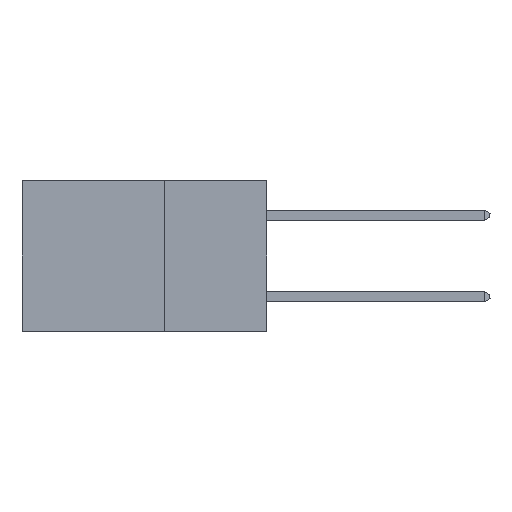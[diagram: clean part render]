
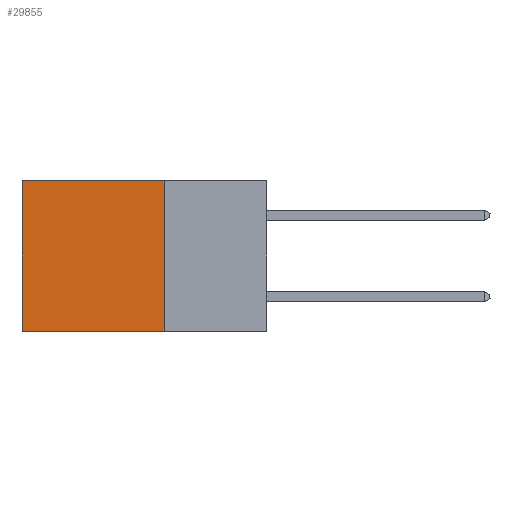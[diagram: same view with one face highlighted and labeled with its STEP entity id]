
A CAD part, left-side view. The second image highlights one B-rep face of the part: STEP entity #29855.
In plain terms, the highlighted planar face has unit normal (-1, 0, 0).
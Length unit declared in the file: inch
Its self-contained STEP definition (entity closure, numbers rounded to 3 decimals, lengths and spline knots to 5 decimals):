
#562 = LINE ( 'NONE', #22025, #26445 ) ;
#1648 = EDGE_CURVE ( 'NONE', #13397, #27911, #10706, .T. ) ;
#1981 = VECTOR ( 'NONE', #32892, 39.37008 ) ;
#3387 = DIRECTION ( 'NONE',  ( 0., 0., -1. ) ) ;
#3437 = CARTESIAN_POINT ( 'NONE',  ( 0.2875, 0.25, 0. ) ) ;
#3974 = DIRECTION ( 'NONE',  ( 0., 1., 0. ) ) ;
#5777 = DIRECTION ( 'NONE',  ( 0., 0., -1. ) ) ;
#6003 = ORIENTED_EDGE ( 'NONE', *, *, #9754, .T. ) ;
#8329 = DIRECTION ( 'NONE',  ( 1., 0., 0. ) ) ;
#9754 = EDGE_CURVE ( 'NONE', #31652, #13397, #562, .T. ) ;
#9827 = CARTESIAN_POINT ( 'NONE',  ( 0.2875, 0.25, -0.37 ) ) ;
#10706 = LINE ( 'NONE', #31030, #23115 ) ;
#11102 = EDGE_CURVE ( 'NONE', #31652, #31467, #21652, .T. ) ;
#11314 = CARTESIAN_POINT ( 'NONE',  ( 0.2875, 0.25, 0. ) ) ;
#12085 = CARTESIAN_POINT ( 'NONE',  ( 0.2875, 0.6, 0. ) ) ;
#13310 = PLANE ( 'NONE',  #28039 ) ;
#13397 = VERTEX_POINT ( 'NONE', #12085 ) ;
#15890 = LINE ( 'NONE', #9827, #1981 ) ;
#16212 = CARTESIAN_POINT ( 'NONE',  ( 0.2875, 0.25, -0.37 ) ) ;
#19039 = EDGE_LOOP ( 'NONE', ( #20692, #30861, #22004, #6003 ) ) ;
#20692 = ORIENTED_EDGE ( 'NONE', *, *, #1648, .T. ) ;
#21652 = LINE ( 'NONE', #23696, #32427 ) ;
#22004 = ORIENTED_EDGE ( 'NONE', *, *, #11102, .F. ) ;
#22025 = CARTESIAN_POINT ( 'NONE',  ( 0.2875, 0.25, 0. ) ) ;
#23115 = VECTOR ( 'NONE', #3387, 39.37008 ) ;
#23696 = CARTESIAN_POINT ( 'NONE',  ( 0.2875, 0.25, 0. ) ) ;
#24284 = CARTESIAN_POINT ( 'NONE',  ( 0.2875, 0.6, -0.37 ) ) ;
#26144 = DIRECTION ( 'NONE',  ( 0., 0., -1. ) ) ;
#26445 = VECTOR ( 'NONE', #3974, 39.37008 ) ;
#27911 = VERTEX_POINT ( 'NONE', #24284 ) ;
#28039 = AXIS2_PLACEMENT_3D ( 'NONE', #3437, #8329, #26144 ) ;
#28749 = EDGE_CURVE ( 'NONE', #31467, #27911, #15890, .T. ) ;
#29855 = ADVANCED_FACE ( 'NONE', ( #30206 ), #13310, .F. ) ;
#30206 = FACE_OUTER_BOUND ( 'NONE', #19039, .T. ) ;
#30861 = ORIENTED_EDGE ( 'NONE', *, *, #28749, .F. ) ;
#31030 = CARTESIAN_POINT ( 'NONE',  ( 0.2875, 0.6, 0. ) ) ;
#31467 = VERTEX_POINT ( 'NONE', #16212 ) ;
#31652 = VERTEX_POINT ( 'NONE', #11314 ) ;
#32427 = VECTOR ( 'NONE', #5777, 39.37008 ) ;
#32892 = DIRECTION ( 'NONE',  ( 0., 1., 0. ) ) ;
